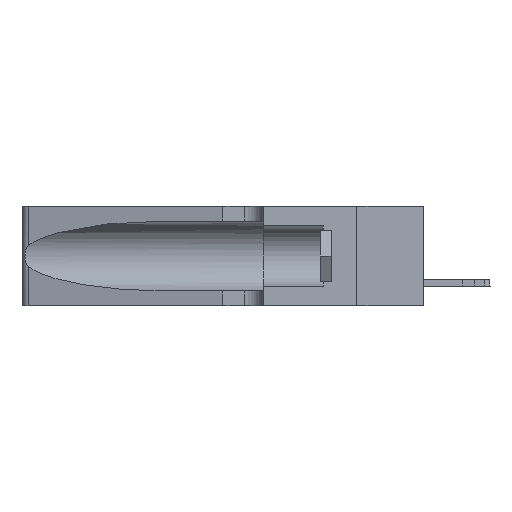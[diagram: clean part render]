
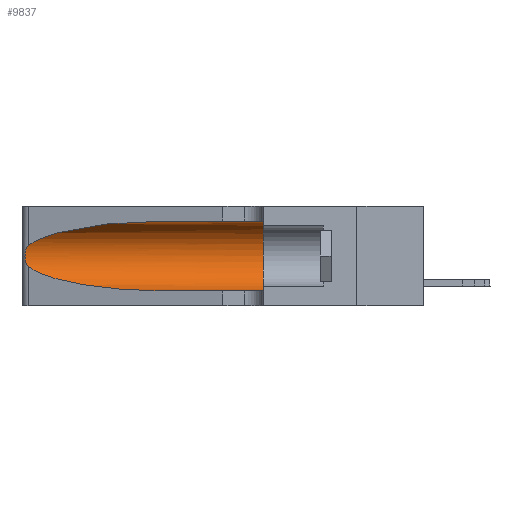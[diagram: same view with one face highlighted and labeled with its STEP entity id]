
A CAD part, left-side view. The second image highlights one B-rep face of the part: STEP entity #9837.
In plain terms, the highlighted cylindrical face has radius 3.308 mm (diameter 6.617 mm), a partial arc.
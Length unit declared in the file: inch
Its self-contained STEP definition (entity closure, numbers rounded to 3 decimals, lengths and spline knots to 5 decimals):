
#235 =( BOUNDED_CURVE ( )  B_SPLINE_CURVE ( 3, ( #32226, #30434, #15226, #2874 ),
 .UNSPECIFIED., .F., .F. ) 
 B_SPLINE_CURVE_WITH_KNOTS ( ( 4, 4 ),
 ( 1.5708, 2.84003 ),
 .UNSPECIFIED. ) 
 CURVE ( )  GEOMETRIC_REPRESENTATION_ITEM ( )  RATIONAL_B_SPLINE_CURVE ( ( 1., 0.87, 0.87, 1. ) ) 
 REPRESENTATION_ITEM ( '' )  );
#421 = CARTESIAN_POINT ( 'NONE',  ( 0.26018, 1.23835, 0.19895 ) ) ;
#1340 = CARTESIAN_POINT ( 'NONE',  ( 0.1305, 0.35, 0.31525 ) ) ;
#1985 = CARTESIAN_POINT ( 'NONE',  ( 0.1305, 1.61858, 0.05475 ) ) ;
#2150 = CARTESIAN_POINT ( 'NONE',  ( 0.2373, 1.15595, 0.08982 ) ) ;
#2559 = CARTESIAN_POINT ( 'NONE',  ( 0.26075, 1.23896, 0.178 ) ) ;
#2563 = EDGE_CURVE ( 'NONE', #22460, #13489, #7995, .T. ) ;
#2874 = CARTESIAN_POINT ( 'NONE',  ( 0.25487, 1.22718, 0.22369 ) ) ;
#3389 = ORIENTED_EDGE ( 'NONE', *, *, #21236, .T. ) ;
#3518 = CARTESIAN_POINT ( 'NONE',  ( 0.25856, 1.23593, 0.16098 ) ) ;
#3848 = VERTEX_POINT ( 'NONE', #20672 ) ;
#5277 = VERTEX_POINT ( 'NONE', #23089 ) ;
#5660 = CARTESIAN_POINT ( 'NONE',  ( 0.25555, 1.22993, 0.14849 ) ) ;
#5821 = CARTESIAN_POINT ( 'NONE',  ( 0.1305, 1.61858, 0.185 ) ) ;
#6086 = B_SPLINE_CURVE_WITH_KNOTS ( 'NONE', 3,
 ( #24464, #27756, #20237, #7862, #22877, #421, #17402, #2559, #7557, #3518, #10585, #18034, #5660, #18266 ),
 .UNSPECIFIED., .F., .F.,
 ( 4, 2, 2, 2, 2, 2, 4 ),
 ( 0., 0.00027, 0.00053, 0.00107, 0.0016, 0.00187, 0.00214 ),
 .UNSPECIFIED. ) ;
#6693 = AXIS2_PLACEMENT_3D ( 'NONE', #5821, #17958, #23594 ) ;
#7557 = CARTESIAN_POINT ( 'NONE',  ( 0.26017, 1.23833, 0.17102 ) ) ;
#7862 = CARTESIAN_POINT ( 'NONE',  ( 0.25787, 1.23484, 0.2124 ) ) ;
#7995 = CIRCLE ( 'NONE', #23221, 0.13025 ) ;
#8519 = EDGE_CURVE ( 'NONE', #5277, #23906, #11909, .T. ) ;
#9140 = ORIENTED_EDGE ( 'NONE', *, *, #13095, .T. ) ;
#9495 = DIRECTION ( 'NONE',  ( 0., 1., 0. ) ) ;
#9604 = DIRECTION ( 'NONE',  ( 0., -1., 0. ) ) ;
#9814 = ORIENTED_EDGE ( 'NONE', *, *, #13241, .T. ) ;
#9837 = ADVANCED_FACE ( 'NONE', ( #11182 ), #15366, .F. ) ;
#10200 = CARTESIAN_POINT ( 'NONE',  ( 0.25487, 1.22718, 0.22369 ) ) ;
#10585 = CARTESIAN_POINT ( 'NONE',  ( 0.25789, 1.23486, 0.15765 ) ) ;
#11182 = FACE_OUTER_BOUND ( 'NONE', #25432, .T. ) ;
#11835 = CARTESIAN_POINT ( 'NONE',  ( 0.1305, 0.72297, 0.05475 ) ) ;
#11909 =( BOUNDED_CURVE ( )  B_SPLINE_CURVE ( 3, ( #26910, #2150, #19206, #11835 ),
 .UNSPECIFIED., .F., .F. ) 
 B_SPLINE_CURVE_WITH_KNOTS ( ( 4, 4 ),
 ( 3.44316, 4.71239 ),
 .UNSPECIFIED. ) 
 CURVE ( )  GEOMETRIC_REPRESENTATION_ITEM ( )  RATIONAL_B_SPLINE_CURVE ( ( 1., 0.87, 0.87, 1. ) ) 
 REPRESENTATION_ITEM ( '' )  );
#11992 = DIRECTION ( 'NONE',  ( 0., 0., 1. ) ) ;
#12062 = CARTESIAN_POINT ( 'NONE',  ( 0.1305, 1.61858, 0.31525 ) ) ;
#13095 = EDGE_CURVE ( 'NONE', #31746, #5277, #6086, .T. ) ;
#13241 = EDGE_CURVE ( 'NONE', #23906, #13489, #24217, .T. ) ;
#13489 = VERTEX_POINT ( 'NONE', #28542 ) ;
#13870 = ORIENTED_EDGE ( 'NONE', *, *, #8519, .T. ) ;
#14563 = ORIENTED_EDGE ( 'NONE', *, *, #2563, .F. ) ;
#15226 = CARTESIAN_POINT ( 'NONE',  ( 0.2373, 1.15595, 0.28018 ) ) ;
#15366 = CYLINDRICAL_SURFACE ( 'NONE', #6693, 0.13025 ) ;
#16823 = EDGE_CURVE ( 'NONE', #3848, #22460, #28097, .T. ) ;
#17402 = CARTESIAN_POINT ( 'NONE',  ( 0.26075, 1.23896, 0.19203 ) ) ;
#17958 = DIRECTION ( 'NONE',  ( 0., -1., 0. ) ) ;
#18034 = CARTESIAN_POINT ( 'NONE',  ( 0.25639, 1.23186, 0.15144 ) ) ;
#18266 = CARTESIAN_POINT ( 'NONE',  ( 0.25487, 1.22718, 0.14631 ) ) ;
#19206 = CARTESIAN_POINT ( 'NONE',  ( 0.18966, 0.96281, 0.05475 ) ) ;
#20237 = CARTESIAN_POINT ( 'NONE',  ( 0.25639, 1.23184, 0.21858 ) ) ;
#20672 = CARTESIAN_POINT ( 'NONE',  ( 0.1305, 0.72297, 0.31525 ) ) ;
#21236 = EDGE_CURVE ( 'NONE', #3848, #31746, #235, .T. ) ;
#21393 = VECTOR ( 'NONE', #30071, 39.37008 ) ;
#21711 = CARTESIAN_POINT ( 'NONE',  ( 0.1305, 0.72297, 0.05475 ) ) ;
#22460 = VERTEX_POINT ( 'NONE', #1340 ) ;
#22597 = VECTOR ( 'NONE', #9604, 39.37008 ) ;
#22877 = CARTESIAN_POINT ( 'NONE',  ( 0.25854, 1.2359, 0.20912 ) ) ;
#23089 = CARTESIAN_POINT ( 'NONE',  ( 0.25487, 1.22718, 0.14631 ) ) ;
#23221 = AXIS2_PLACEMENT_3D ( 'NONE', #24413, #9495, #11992 ) ;
#23594 = DIRECTION ( 'NONE',  ( 0., 0., -1. ) ) ;
#23906 = VERTEX_POINT ( 'NONE', #21711 ) ;
#24217 = LINE ( 'NONE', #1985, #22597 ) ;
#24413 = CARTESIAN_POINT ( 'NONE',  ( 0.1305, 0.35, 0.185 ) ) ;
#24464 = CARTESIAN_POINT ( 'NONE',  ( 0.25487, 1.22718, 0.22369 ) ) ;
#25432 = EDGE_LOOP ( 'NONE', ( #3389, #9140, #13870, #9814, #14563, #32395 ) ) ;
#26910 = CARTESIAN_POINT ( 'NONE',  ( 0.25487, 1.22718, 0.14631 ) ) ;
#27756 = CARTESIAN_POINT ( 'NONE',  ( 0.25555, 1.22994, 0.2215 ) ) ;
#28097 = LINE ( 'NONE', #12062, #21393 ) ;
#28542 = CARTESIAN_POINT ( 'NONE',  ( 0.1305, 0.35, 0.05475 ) ) ;
#30071 = DIRECTION ( 'NONE',  ( 0., -1., 0. ) ) ;
#30434 = CARTESIAN_POINT ( 'NONE',  ( 0.18966, 0.96281, 0.31525 ) ) ;
#31746 = VERTEX_POINT ( 'NONE', #10200 ) ;
#32226 = CARTESIAN_POINT ( 'NONE',  ( 0.1305, 0.72297, 0.31525 ) ) ;
#32395 = ORIENTED_EDGE ( 'NONE', *, *, #16823, .F. ) ;
